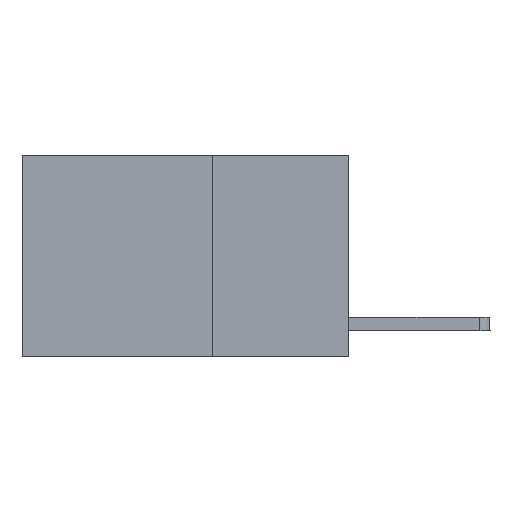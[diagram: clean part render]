
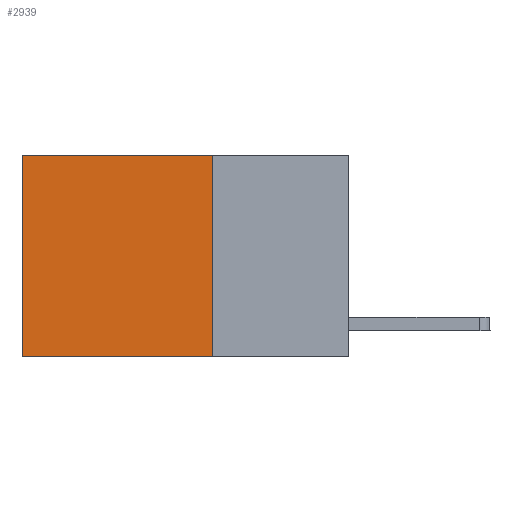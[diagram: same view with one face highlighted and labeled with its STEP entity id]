
A CAD part, left-side view. The second image highlights one B-rep face of the part: STEP entity #2939.
In plain terms, the highlighted planar face has unit normal (-1, 0, 0).
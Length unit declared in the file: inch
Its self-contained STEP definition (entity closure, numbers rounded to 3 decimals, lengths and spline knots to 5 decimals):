
#125 = CARTESIAN_POINT ( 'NONE',  ( 0.2625, 0.25, 0. ) ) ;
#258 = ORIENTED_EDGE ( 'NONE', *, *, #9321, .F. ) ;
#878 = DIRECTION ( 'NONE',  ( 1., 0., 0. ) ) ;
#1203 = LINE ( 'NONE', #3545, #2221 ) ;
#1223 = DIRECTION ( 'NONE',  ( 0., 1., 0. ) ) ;
#1270 = VERTEX_POINT ( 'NONE', #1577 ) ;
#1569 = EDGE_CURVE ( 'NONE', #4578, #3377, #1203, .T. ) ;
#1577 = CARTESIAN_POINT ( 'NONE',  ( 0.2625, 0.25, 0. ) ) ;
#2221 = VECTOR ( 'NONE', #5013, 39.37008 ) ;
#2589 = LINE ( 'NONE', #9545, #5698 ) ;
#2702 = LINE ( 'NONE', #8960, #7915 ) ;
#2939 = ADVANCED_FACE ( 'NONE', ( #9267 ), #7059, .F. ) ;
#2972 = DIRECTION ( 'NONE',  ( 0., 0., -1. ) ) ;
#3227 = DIRECTION ( 'NONE',  ( 0., 0., -1. ) ) ;
#3243 = ORIENTED_EDGE ( 'NONE', *, *, #7040, .T. ) ;
#3290 = EDGE_LOOP ( 'NONE', ( #3493, #7967, #258, #3243 ) ) ;
#3377 = VERTEX_POINT ( 'NONE', #6094 ) ;
#3460 = DIRECTION ( 'NONE',  ( 0., 1., 0. ) ) ;
#3493 = ORIENTED_EDGE ( 'NONE', *, *, #1569, .T. ) ;
#3545 = CARTESIAN_POINT ( 'NONE',  ( 0.2625, 0.6, 0. ) ) ;
#4032 = VERTEX_POINT ( 'NONE', #7852 ) ;
#4293 = VECTOR ( 'NONE', #2972, 39.37008 ) ;
#4578 = VERTEX_POINT ( 'NONE', #5817 ) ;
#4965 = LINE ( 'NONE', #8048, #4293 ) ;
#5013 = DIRECTION ( 'NONE',  ( 0., 0., -1. ) ) ;
#5211 = EDGE_CURVE ( 'NONE', #4032, #3377, #2589, .T. ) ;
#5698 = VECTOR ( 'NONE', #3460, 39.37008 ) ;
#5817 = CARTESIAN_POINT ( 'NONE',  ( 0.2625, 0.6, 0. ) ) ;
#6094 = CARTESIAN_POINT ( 'NONE',  ( 0.2625, 0.6, -0.37 ) ) ;
#7040 = EDGE_CURVE ( 'NONE', #1270, #4578, #2702, .T. ) ;
#7059 = PLANE ( 'NONE',  #7721 ) ;
#7721 = AXIS2_PLACEMENT_3D ( 'NONE', #125, #878, #3227 ) ;
#7852 = CARTESIAN_POINT ( 'NONE',  ( 0.2625, 0.25, -0.37 ) ) ;
#7915 = VECTOR ( 'NONE', #1223, 39.37008 ) ;
#7967 = ORIENTED_EDGE ( 'NONE', *, *, #5211, .F. ) ;
#8048 = CARTESIAN_POINT ( 'NONE',  ( 0.2625, 0.25, 0. ) ) ;
#8960 = CARTESIAN_POINT ( 'NONE',  ( 0.2625, 0.25, 0. ) ) ;
#9267 = FACE_OUTER_BOUND ( 'NONE', #3290, .T. ) ;
#9321 = EDGE_CURVE ( 'NONE', #1270, #4032, #4965, .T. ) ;
#9545 = CARTESIAN_POINT ( 'NONE',  ( 0.2625, 0.25, -0.37 ) ) ;
